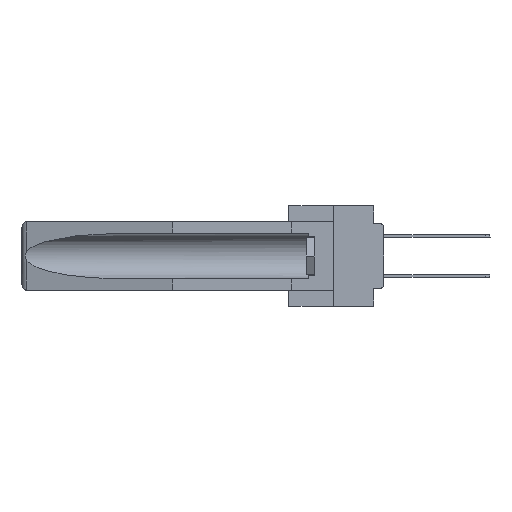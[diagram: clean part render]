
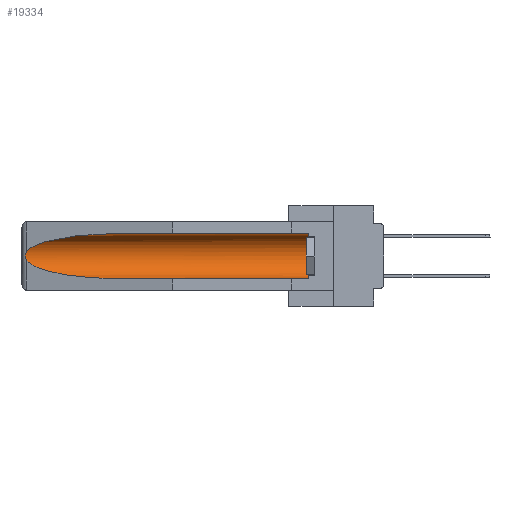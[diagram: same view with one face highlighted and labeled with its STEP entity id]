
A CAD part, left-side view. The second image highlights one B-rep face of the part: STEP entity #19334.
In plain terms, the highlighted cylindrical face has radius 2.857 mm (diameter 5.715 mm), a partial arc.
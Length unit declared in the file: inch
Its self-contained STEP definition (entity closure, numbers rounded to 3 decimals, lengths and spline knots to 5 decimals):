
#419 = CARTESIAN_POINT ( 'NONE',  ( 0.26537, 1.52718, -0.14972 ) ) ;
#1439 = CARTESIAN_POINT ( 'NONE',  ( 0.155, 0.126, -0.059 ) ) ;
#2938 = CARTESIAN_POINT ( 'NONE',  ( 0.26597, 1.52961, -0.15275 ) ) ;
#4059 = B_SPLINE_CURVE_WITH_KNOTS ( 'NONE', 3,
 ( #419, #2938, #21585, #21258, #13546, #24190, #23856, #21138, #26357, #5683 ),
 .UNSPECIFIED., .F., .F.,
 ( 4, 2, 2, 2, 4 ),
 ( 0., 0.00029, 0.00058, 0.00087, 0.00117 ),
 .UNSPECIFIED. ) ;
#4192 = VERTEX_POINT ( 'NONE', #14882 ) ;
#4322 = ORIENTED_EDGE ( 'NONE', *, *, #7882, .T. ) ;
#4645 = VECTOR ( 'NONE', #15344, 39.37008 ) ;
#4854 = CYLINDRICAL_SURFACE ( 'NONE', #11804, 0.1125 ) ;
#5197 = CARTESIAN_POINT ( 'NONE',  ( 0.26537, 1.52718, -0.19328 ) ) ;
#5683 = CARTESIAN_POINT ( 'NONE',  ( 0.26537, 1.52718, -0.19328 ) ) ;
#6560 = CARTESIAN_POINT ( 'NONE',  ( 0.155, -0.30754, -0.284 ) ) ;
#6590 = CARTESIAN_POINT ( 'NONE',  ( 0.155, 1.07973, -0.284 ) ) ;
#6837 = EDGE_CURVE ( 'NONE', #4192, #11831, #10092, .T. ) ;
#6962 = VECTOR ( 'NONE', #32291, 39.37008 ) ;
#6997 = CARTESIAN_POINT ( 'NONE',  ( 0.155, 0.126, -0.1715 ) ) ;
#7311 = VERTEX_POINT ( 'NONE', #28152 ) ;
#7882 = EDGE_CURVE ( 'NONE', #11831, #31594, #4059, .T. ) ;
#7899 = LINE ( 'NONE', #22939, #4645 ) ;
#8082 = DIRECTION ( 'NONE',  ( 0., 1., 0. ) ) ;
#9609 = ORIENTED_EDGE ( 'NONE', *, *, #31508, .T. ) ;
#9930 = ORIENTED_EDGE ( 'NONE', *, *, #18305, .F. ) ;
#9961 = VERTEX_POINT ( 'NONE', #6590 ) ;
#10092 =( BOUNDED_CURVE ( )  B_SPLINE_CURVE ( 3, ( #12212, #16990, #20045, #22645 ),
 .UNSPECIFIED., .F., .F. ) 
 B_SPLINE_CURVE_WITH_KNOTS ( ( 4, 4 ),
 ( 4.71239, 6.08839 ),
 .UNSPECIFIED. ) 
 CURVE ( )  GEOMETRIC_REPRESENTATION_ITEM ( )  RATIONAL_B_SPLINE_CURVE ( ( 1., 0.848, 0.848, 1. ) ) 
 REPRESENTATION_ITEM ( '' )  );
#10168 = EDGE_CURVE ( 'NONE', #25836, #4192, #7899, .T. ) ;
#11804 = AXIS2_PLACEMENT_3D ( 'NONE', #31218, #8082, #28841 ) ;
#11818 = CIRCLE ( 'NONE', #27221, 0.1125 ) ;
#11831 = VERTEX_POINT ( 'NONE', #13302 ) ;
#12210 = FACE_OUTER_BOUND ( 'NONE', #29985, .T. ) ;
#12212 = CARTESIAN_POINT ( 'NONE',  ( 0.155, 1.07973, -0.059 ) ) ;
#13054 = CARTESIAN_POINT ( 'NONE',  ( 0.155, 1.07973, -0.284 ) ) ;
#13302 = CARTESIAN_POINT ( 'NONE',  ( 0.26537, 1.52718, -0.14972 ) ) ;
#13546 = CARTESIAN_POINT ( 'NONE',  ( 0.2675, 1.53308, -0.16763 ) ) ;
#14428 = DIRECTION ( 'NONE',  ( 0., -1., 0. ) ) ;
#14682 = ORIENTED_EDGE ( 'NONE', *, *, #26163, .T. ) ;
#14882 = CARTESIAN_POINT ( 'NONE',  ( 0.155, 1.07973, -0.059 ) ) ;
#15201 = CARTESIAN_POINT ( 'NONE',  ( 0.26537, 1.52718, -0.19328 ) ) ;
#15344 = DIRECTION ( 'NONE',  ( 0., 1., 0. ) ) ;
#15792 = ORIENTED_EDGE ( 'NONE', *, *, #10168, .T. ) ;
#16990 = CARTESIAN_POINT ( 'NONE',  ( 0.21114, 1.30732, -0.059 ) ) ;
#18176 = CARTESIAN_POINT ( 'NONE',  ( 0.21114, 1.30732, -0.284 ) ) ;
#18305 = EDGE_CURVE ( 'NONE', #7311, #9961, #28093, .T. ) ;
#19334 = ADVANCED_FACE ( 'NONE', ( #12210 ), #4854, .F. ) ;
#20045 = CARTESIAN_POINT ( 'NONE',  ( 0.25451, 1.48313, -0.09465 ) ) ;
#21138 = CARTESIAN_POINT ( 'NONE',  ( 0.26655, 1.53094, -0.18657 ) ) ;
#21258 = CARTESIAN_POINT ( 'NONE',  ( 0.2673, 1.5327, -0.16383 ) ) ;
#21585 = CARTESIAN_POINT ( 'NONE',  ( 0.26654, 1.53092, -0.15636 ) ) ;
#22645 = CARTESIAN_POINT ( 'NONE',  ( 0.26537, 1.52718, -0.14972 ) ) ;
#22939 = CARTESIAN_POINT ( 'NONE',  ( 0.155, -0.30754, -0.059 ) ) ;
#23595 = ORIENTED_EDGE ( 'NONE', *, *, #6837, .T. ) ;
#23856 = CARTESIAN_POINT ( 'NONE',  ( 0.2673, 1.53269, -0.17917 ) ) ;
#24190 = CARTESIAN_POINT ( 'NONE',  ( 0.2675, 1.53308, -0.17534 ) ) ;
#25133 =( BOUNDED_CURVE ( )  B_SPLINE_CURVE ( 3, ( #5197, #25875, #18176, #13054 ),
 .UNSPECIFIED., .F., .T. ) 
 B_SPLINE_CURVE_WITH_KNOTS ( ( 4, 4 ),
 ( 0.1948, 1.5708 ),
 .UNSPECIFIED. ) 
 CURVE ( )  GEOMETRIC_REPRESENTATION_ITEM ( )  RATIONAL_B_SPLINE_CURVE ( ( 1., 0.848, 0.848, 1. ) ) 
 REPRESENTATION_ITEM ( '' )  );
#25836 = VERTEX_POINT ( 'NONE', #1439 ) ;
#25875 = CARTESIAN_POINT ( 'NONE',  ( 0.25451, 1.48313, -0.24835 ) ) ;
#26163 = EDGE_CURVE ( 'NONE', #31594, #9961, #25133, .T. ) ;
#26357 = CARTESIAN_POINT ( 'NONE',  ( 0.26597, 1.5296, -0.19026 ) ) ;
#27221 = AXIS2_PLACEMENT_3D ( 'NONE', #6997, #14428, #27774 ) ;
#27774 = DIRECTION ( 'NONE',  ( 0., 0., 1. ) ) ;
#28093 = LINE ( 'NONE', #6560, #6962 ) ;
#28152 = CARTESIAN_POINT ( 'NONE',  ( 0.155, 0.126, -0.284 ) ) ;
#28841 = DIRECTION ( 'NONE',  ( 0., 0., 1. ) ) ;
#29985 = EDGE_LOOP ( 'NONE', ( #23595, #4322, #14682, #9930, #9609, #15792 ) ) ;
#31218 = CARTESIAN_POINT ( 'NONE',  ( 0.155, -0.30754, -0.1715 ) ) ;
#31508 = EDGE_CURVE ( 'NONE', #7311, #25836, #11818, .T. ) ;
#31594 = VERTEX_POINT ( 'NONE', #15201 ) ;
#32291 = DIRECTION ( 'NONE',  ( 0., 1., 0. ) ) ;
